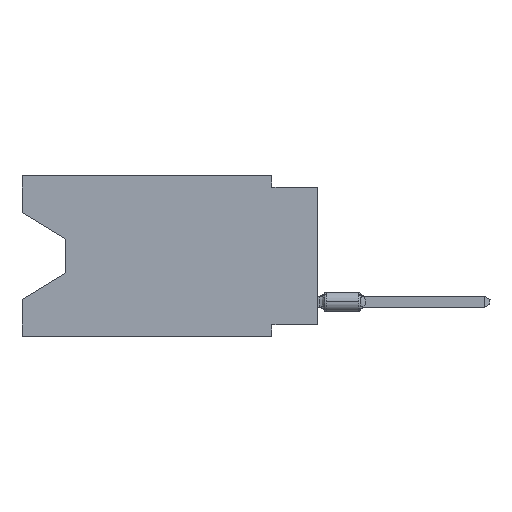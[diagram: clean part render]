
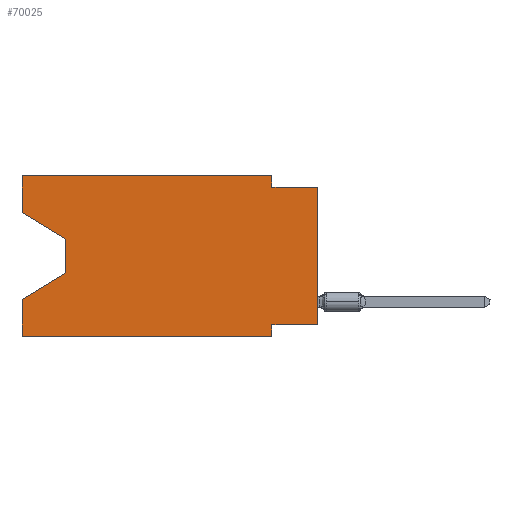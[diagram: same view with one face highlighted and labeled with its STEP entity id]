
A CAD part, left-side view. The second image highlights one B-rep face of the part: STEP entity #70025.
In plain terms, the highlighted planar face has unit normal (-1, 0, 0).
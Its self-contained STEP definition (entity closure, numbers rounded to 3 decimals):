
#345 = EDGE_CURVE ( 'NONE', #35653, #48274, #36303, .T. ) ;
#590 = ORIENTED_EDGE ( 'NONE', *, *, #78275, .F. ) ;
#1306 = CARTESIAN_POINT ( 'NONE',  ( 0., 13.97, -5.385 ) ) ;
#1983 = VECTOR ( 'NONE', #47605, 1000. ) ;
#2797 = EDGE_CURVE ( 'NONE', #48274, #53245, #60453, .T. ) ;
#3222 = DIRECTION ( 'NONE',  ( 0., 0., -1. ) ) ;
#5365 = CARTESIAN_POINT ( 'NONE',  ( 0., 16.383, 0. ) ) ;
#5989 = ORIENTED_EDGE ( 'NONE', *, *, #62331, .F. ) ;
#6524 = DIRECTION ( 'NONE',  ( 0., -0.855, -0.519 ) ) ;
#7987 = LINE ( 'NONE', #41934, #1983 ) ;
#9616 = CARTESIAN_POINT ( 'NONE',  ( 0., 16.383, -8.89 ) ) ;
#9662 = CARTESIAN_POINT ( 'NONE',  ( 0., 2.54, -8.89 ) ) ;
#9891 = ORIENTED_EDGE ( 'NONE', *, *, #2797, .T. ) ;
#10253 = VERTEX_POINT ( 'NONE', #69749 ) ;
#11509 = EDGE_CURVE ( 'NONE', #78084, #53245, #38022, .T. ) ;
#11895 = VERTEX_POINT ( 'NONE', #43585 ) ;
#12138 = CARTESIAN_POINT ( 'NONE',  ( 0., 0., -0.635 ) ) ;
#13450 = LINE ( 'NONE', #85673, #70756 ) ;
#14245 = LINE ( 'NONE', #55575, #43502 ) ;
#14594 = VERTEX_POINT ( 'NONE', #78629 ) ;
#15108 = CARTESIAN_POINT ( 'NONE',  ( 0., 2.54, -8.255 ) ) ;
#15452 = EDGE_CURVE ( 'NONE', #72002, #35653, #26549, .T. ) ;
#15743 = EDGE_CURVE ( 'NONE', #72002, #11895, #30398, .T. ) ;
#16692 = VECTOR ( 'NONE', #3222, 1000. ) ;
#16889 = DIRECTION ( 'NONE',  ( 0., 0., 1. ) ) ;
#17138 = CARTESIAN_POINT ( 'NONE',  ( 0., 0., -0.635 ) ) ;
#17955 = VECTOR ( 'NONE', #82714, 1000. ) ;
#18606 = CARTESIAN_POINT ( 'NONE',  ( 0., 16.383, -2.038 ) ) ;
#19000 = CARTESIAN_POINT ( 'NONE',  ( 0., 2.54, 0. ) ) ;
#21940 = CARTESIAN_POINT ( 'NONE',  ( 0., 16.383, -8.89 ) ) ;
#23080 = FACE_OUTER_BOUND ( 'NONE', #43605, .T. ) ;
#24515 = DIRECTION ( 'NONE',  ( 0., -1., 0. ) ) ;
#24693 = EDGE_CURVE ( 'NONE', #14594, #52611, #13450, .T. ) ;
#26193 = EDGE_CURVE ( 'NONE', #78084, #54228, #29210, .T. ) ;
#26549 = LINE ( 'NONE', #38743, #79487 ) ;
#26769 = VECTOR ( 'NONE', #16889, 1000. ) ;
#29085 = CARTESIAN_POINT ( 'NONE',  ( 0., 0., -8.255 ) ) ;
#29210 = LINE ( 'NONE', #9616, #17955 ) ;
#30398 = LINE ( 'NONE', #43460, #26769 ) ;
#31060 = LINE ( 'NONE', #84116, #54120 ) ;
#35653 = VERTEX_POINT ( 'NONE', #50882 ) ;
#36303 = LINE ( 'NONE', #62835, #16692 ) ;
#38022 = LINE ( 'NONE', #5365, #49834 ) ;
#38743 = CARTESIAN_POINT ( 'NONE',  ( 0., 16.383, -2.038 ) ) ;
#39268 = ORIENTED_EDGE ( 'NONE', *, *, #72571, .F. ) ;
#39436 = ORIENTED_EDGE ( 'NONE', *, *, #15452, .T. ) ;
#40808 = DIRECTION ( 'NONE',  ( 0., 0., -1. ) ) ;
#41934 = CARTESIAN_POINT ( 'NONE',  ( 0., 2.54, -8.89 ) ) ;
#42130 = VECTOR ( 'NONE', #48250, 1000. ) ;
#43109 = DIRECTION ( 'NONE',  ( 0., 0., -1. ) ) ;
#43460 = CARTESIAN_POINT ( 'NONE',  ( 0., 16.383, 0. ) ) ;
#43502 = VECTOR ( 'NONE', #40808, 1000. ) ;
#43585 = CARTESIAN_POINT ( 'NONE',  ( 0., 16.383, 0. ) ) ;
#43605 = EDGE_LOOP ( 'NONE', ( #39436, #56549, #9891, #58304, #44577, #76891, #39268, #45638, #69059, #5989, #590, #77479 ) ) ;
#44577 = ORIENTED_EDGE ( 'NONE', *, *, #26193, .T. ) ;
#45394 = DIRECTION ( 'NONE',  ( 0., 0., 1. ) ) ;
#45411 = VERTEX_POINT ( 'NONE', #15108 ) ;
#45638 = ORIENTED_EDGE ( 'NONE', *, *, #24693, .T. ) ;
#46081 = DIRECTION ( 'NONE',  ( 0., -1., 0. ) ) ;
#46485 = EDGE_CURVE ( 'NONE', #10253, #52611, #58696, .T. ) ;
#47605 = DIRECTION ( 'NONE',  ( 0., 0., -1. ) ) ;
#48250 = DIRECTION ( 'NONE',  ( 0., 0.855, -0.519 ) ) ;
#48274 = VERTEX_POINT ( 'NONE', #1306 ) ;
#49834 = VECTOR ( 'NONE', #45394, 1000. ) ;
#50882 = CARTESIAN_POINT ( 'NONE',  ( 0., 13.97, -3.505 ) ) ;
#51421 = CARTESIAN_POINT ( 'NONE',  ( 0., 16.383, -6.852 ) ) ;
#52611 = VERTEX_POINT ( 'NONE', #17138 ) ;
#53074 = DIRECTION ( 'NONE',  ( 0., 0., 1. ) ) ;
#53245 = VERTEX_POINT ( 'NONE', #51421 ) ;
#54120 = VECTOR ( 'NONE', #24515, 1000. ) ;
#54228 = VERTEX_POINT ( 'NONE', #9662 ) ;
#55575 = CARTESIAN_POINT ( 'NONE',  ( 0., 2.54, 0. ) ) ;
#56086 = AXIS2_PLACEMENT_3D ( 'NONE', #76164, #63534, #43109 ) ;
#56549 = ORIENTED_EDGE ( 'NONE', *, *, #345, .T. ) ;
#58304 = ORIENTED_EDGE ( 'NONE', *, *, #11509, .F. ) ;
#58696 = LINE ( 'NONE', #12138, #62105 ) ;
#60453 = LINE ( 'NONE', #67811, #42130 ) ;
#62105 = VECTOR ( 'NONE', #46081, 1000. ) ;
#62331 = EDGE_CURVE ( 'NONE', #84437, #10253, #14245, .T. ) ;
#62835 = CARTESIAN_POINT ( 'NONE',  ( 0., 13.97, -3.505 ) ) ;
#63534 = DIRECTION ( 'NONE',  ( 1., 0., 0. ) ) ;
#63766 = EDGE_CURVE ( 'NONE', #45411, #54228, #7987, .T. ) ;
#67811 = CARTESIAN_POINT ( 'NONE',  ( 0., 13.97, -5.385 ) ) ;
#69059 = ORIENTED_EDGE ( 'NONE', *, *, #46485, .F. ) ;
#69749 = CARTESIAN_POINT ( 'NONE',  ( 0., 2.54, -0.635 ) ) ;
#70025 = ADVANCED_FACE ( 'NONE', ( #23080 ), #70048, .F. ) ;
#70048 = PLANE ( 'NONE',  #56086 ) ;
#70705 = DIRECTION ( 'NONE',  ( 0., 1., 0. ) ) ;
#70756 = VECTOR ( 'NONE', #53074, 1000. ) ;
#72002 = VERTEX_POINT ( 'NONE', #18606 ) ;
#72571 = EDGE_CURVE ( 'NONE', #14594, #45411, #77248, .T. ) ;
#76164 = CARTESIAN_POINT ( 'NONE',  ( 0., 16.383, 0. ) ) ;
#76891 = ORIENTED_EDGE ( 'NONE', *, *, #63766, .F. ) ;
#77248 = LINE ( 'NONE', #29085, #81212 ) ;
#77479 = ORIENTED_EDGE ( 'NONE', *, *, #15743, .F. ) ;
#78084 = VERTEX_POINT ( 'NONE', #21940 ) ;
#78275 = EDGE_CURVE ( 'NONE', #11895, #84437, #31060, .T. ) ;
#78629 = CARTESIAN_POINT ( 'NONE',  ( 0., 0., -8.255 ) ) ;
#79487 = VECTOR ( 'NONE', #6524, 1000. ) ;
#81212 = VECTOR ( 'NONE', #70705, 1000. ) ;
#82714 = DIRECTION ( 'NONE',  ( 0., -1., 0. ) ) ;
#84116 = CARTESIAN_POINT ( 'NONE',  ( 0., 16.383, 0. ) ) ;
#84437 = VERTEX_POINT ( 'NONE', #19000 ) ;
#85673 = CARTESIAN_POINT ( 'NONE',  ( 0., 0., 0. ) ) ;
